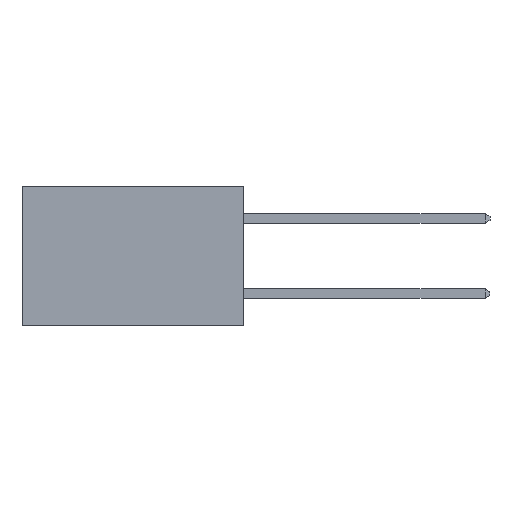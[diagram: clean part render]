
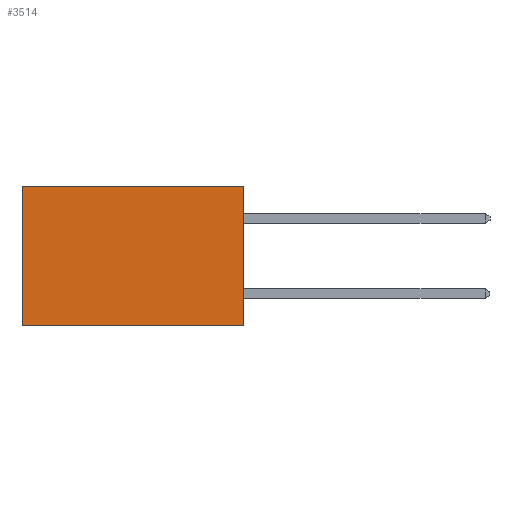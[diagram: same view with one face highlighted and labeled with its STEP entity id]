
A CAD part, left-side view. The second image highlights one B-rep face of the part: STEP entity #3514.
In plain terms, the highlighted planar face has unit normal (-1, 0, 0).
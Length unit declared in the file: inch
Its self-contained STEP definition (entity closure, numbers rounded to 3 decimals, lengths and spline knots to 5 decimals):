
#32 = CARTESIAN_POINT ( 'NONE',  ( 0.277, 0., -0.37 ) ) ;
#118 = ORIENTED_EDGE ( 'NONE', *, *, #4232, .T. ) ;
#165 = ORIENTED_EDGE ( 'NONE', *, *, #6034, .F. ) ;
#217 = ORIENTED_EDGE ( 'NONE', *, *, #1152, .F. ) ;
#377 = ORIENTED_EDGE ( 'NONE', *, *, #4331, .T. ) ;
#409 = LINE ( 'NONE', #3645, #1917 ) ;
#743 = VERTEX_POINT ( 'NONE', #3075 ) ;
#748 = VECTOR ( 'NONE', #6077, 39.37008 ) ;
#792 = VERTEX_POINT ( 'NONE', #5451 ) ;
#1152 = EDGE_CURVE ( 'NONE', #792, #6772, #2800, .T. ) ;
#1323 = EDGE_LOOP ( 'NONE', ( #118, #165, #217, #377 ) ) ;
#1622 = VECTOR ( 'NONE', #6483, 39.37008 ) ;
#1821 = DIRECTION ( 'NONE',  ( 0., 0., -1. ) ) ;
#1829 = DIRECTION ( 'NONE',  ( 1., 0., 0. ) ) ;
#1831 = PLANE ( 'NONE',  #2835 ) ;
#1917 = VECTOR ( 'NONE', #3735, 39.37008 ) ;
#2463 = CARTESIAN_POINT ( 'NONE',  ( 0.277, 0., -0.37 ) ) ;
#2627 = VECTOR ( 'NONE', #7366, 39.37008 ) ;
#2800 = LINE ( 'NONE', #7126, #2627 ) ;
#2835 = AXIS2_PLACEMENT_3D ( 'NONE', #2463, #1829, #1821 ) ;
#3075 = CARTESIAN_POINT ( 'NONE',  ( 0.277, 0.59, 0. ) ) ;
#3177 = VERTEX_POINT ( 'NONE', #4137 ) ;
#3514 = ADVANCED_FACE ( 'NONE', ( #6147 ), #1831, .F. ) ;
#3645 = CARTESIAN_POINT ( 'NONE',  ( 0.277, 0., 0. ) ) ;
#3735 = DIRECTION ( 'NONE',  ( 0., 1., 0. ) ) ;
#4137 = CARTESIAN_POINT ( 'NONE',  ( 0.277, 0.59, -0.37 ) ) ;
#4232 = EDGE_CURVE ( 'NONE', #743, #3177, #4665, .T. ) ;
#4331 = EDGE_CURVE ( 'NONE', #792, #743, #409, .T. ) ;
#4665 = LINE ( 'NONE', #6485, #1622 ) ;
#5451 = CARTESIAN_POINT ( 'NONE',  ( 0.277, 0., 0. ) ) ;
#6034 = EDGE_CURVE ( 'NONE', #6772, #3177, #7056, .T. ) ;
#6077 = DIRECTION ( 'NONE',  ( 0., 1., 0. ) ) ;
#6147 = FACE_OUTER_BOUND ( 'NONE', #1323, .T. ) ;
#6187 = CARTESIAN_POINT ( 'NONE',  ( 0.277, 0., -0.37 ) ) ;
#6483 = DIRECTION ( 'NONE',  ( 0., 0., -1. ) ) ;
#6485 = CARTESIAN_POINT ( 'NONE',  ( 0.277, 0.59, -0.37 ) ) ;
#6772 = VERTEX_POINT ( 'NONE', #6187 ) ;
#7056 = LINE ( 'NONE', #32, #748 ) ;
#7126 = CARTESIAN_POINT ( 'NONE',  ( 0.277, 0., -0.37 ) ) ;
#7366 = DIRECTION ( 'NONE',  ( 0., 0., -1. ) ) ;
